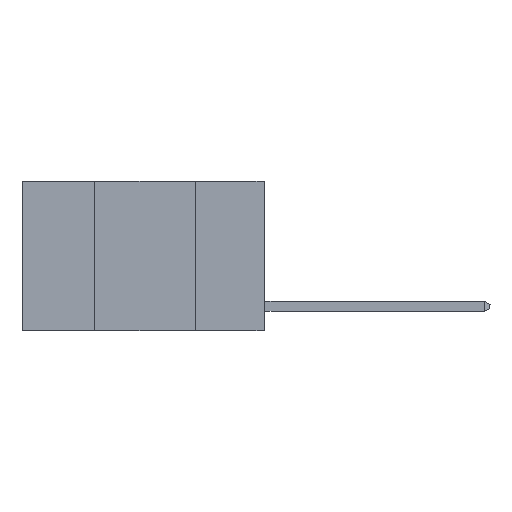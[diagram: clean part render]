
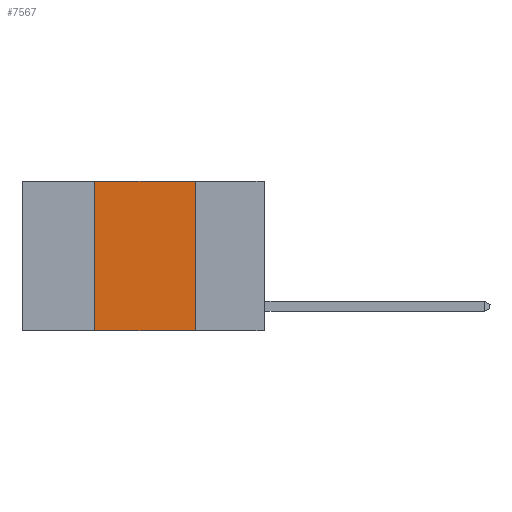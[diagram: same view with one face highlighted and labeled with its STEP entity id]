
A CAD part, left-side view. The second image highlights one B-rep face of the part: STEP entity #7567.
In plain terms, the highlighted planar face has unit normal (-1, 0, 0).
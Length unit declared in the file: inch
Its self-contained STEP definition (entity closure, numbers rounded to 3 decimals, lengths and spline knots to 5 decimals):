
#549 = VECTOR ( 'NONE', #11709, 39.37008 ) ;
#1205 = DIRECTION ( 'NONE',  ( 1., 0., 0. ) ) ;
#1614 = VERTEX_POINT ( 'NONE', #9150 ) ;
#1653 = DIRECTION ( 'NONE',  ( 0., 0., 1. ) ) ;
#2008 = VERTEX_POINT ( 'NONE', #11075 ) ;
#2215 = DIRECTION ( 'NONE',  ( 0., -1., 0. ) ) ;
#2274 = LINE ( 'NONE', #7529, #11091 ) ;
#2331 = CARTESIAN_POINT ( 'NONE',  ( 0., 0.17, 0. ) ) ;
#2342 = PLANE ( 'NONE',  #12506 ) ;
#2372 = VERTEX_POINT ( 'NONE', #3950 ) ;
#2811 = EDGE_LOOP ( 'NONE', ( #7947, #4385, #7233, #4423 ) ) ;
#3348 = DIRECTION ( 'NONE',  ( 0., 0., -1. ) ) ;
#3782 = LINE ( 'NONE', #6890, #5615 ) ;
#3950 = CARTESIAN_POINT ( 'NONE',  ( 0., 0.42, 0. ) ) ;
#4228 = EDGE_CURVE ( 'NONE', #2372, #1614, #3782, .T. ) ;
#4385 = ORIENTED_EDGE ( 'NONE', *, *, #4228, .F. ) ;
#4423 = ORIENTED_EDGE ( 'NONE', *, *, #8513, .T. ) ;
#5174 = VECTOR ( 'NONE', #1653, 39.37008 ) ;
#5615 = VECTOR ( 'NONE', #7897, 39.37008 ) ;
#6890 = CARTESIAN_POINT ( 'NONE',  ( 0., 0.6, 0. ) ) ;
#7233 = ORIENTED_EDGE ( 'NONE', *, *, #10489, .F. ) ;
#7529 = CARTESIAN_POINT ( 'NONE',  ( 0., 0.6, -0.37 ) ) ;
#7531 = FACE_OUTER_BOUND ( 'NONE', #2811, .T. ) ;
#7567 = ADVANCED_FACE ( 'NONE', ( #7531 ), #2342, .F. ) ;
#7585 = CARTESIAN_POINT ( 'NONE',  ( 0., 0.42, 0. ) ) ;
#7897 = DIRECTION ( 'NONE',  ( 0., -1., 0. ) ) ;
#7947 = ORIENTED_EDGE ( 'NONE', *, *, #12190, .F. ) ;
#8513 = EDGE_CURVE ( 'NONE', #2008, #12022, #2274, .T. ) ;
#8574 = CARTESIAN_POINT ( 'NONE',  ( 0., 0.6, 0. ) ) ;
#8752 = LINE ( 'NONE', #7585, #5174 ) ;
#9150 = CARTESIAN_POINT ( 'NONE',  ( 0., 0.17, 0. ) ) ;
#10489 = EDGE_CURVE ( 'NONE', #2008, #2372, #8752, .T. ) ;
#10979 = CARTESIAN_POINT ( 'NONE',  ( 0., 0.17, -0.37 ) ) ;
#11075 = CARTESIAN_POINT ( 'NONE',  ( 0., 0.42, -0.37 ) ) ;
#11091 = VECTOR ( 'NONE', #2215, 39.37008 ) ;
#11315 = LINE ( 'NONE', #2331, #549 ) ;
#11709 = DIRECTION ( 'NONE',  ( 0., 0., -1. ) ) ;
#12022 = VERTEX_POINT ( 'NONE', #10979 ) ;
#12190 = EDGE_CURVE ( 'NONE', #1614, #12022, #11315, .T. ) ;
#12506 = AXIS2_PLACEMENT_3D ( 'NONE', #8574, #1205, #3348 ) ;
